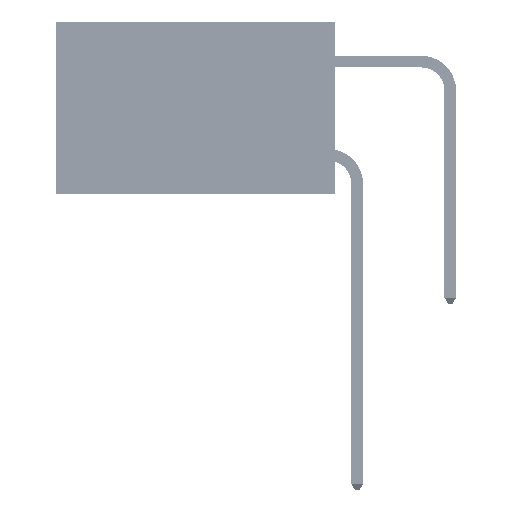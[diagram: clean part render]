
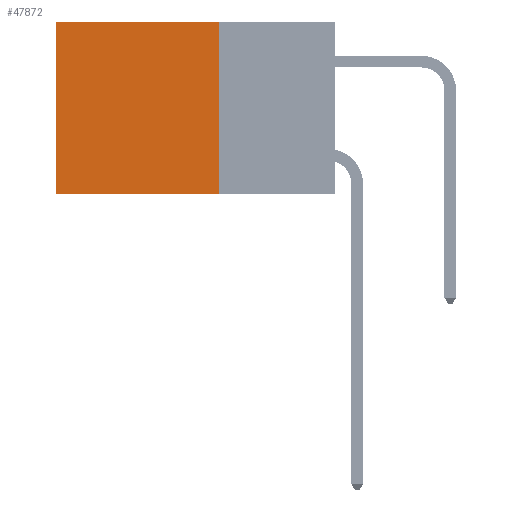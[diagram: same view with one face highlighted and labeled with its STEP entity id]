
A CAD part, left-side view. The second image highlights one B-rep face of the part: STEP entity #47872.
In plain terms, the highlighted planar face has unit normal (-1, 0, 0).
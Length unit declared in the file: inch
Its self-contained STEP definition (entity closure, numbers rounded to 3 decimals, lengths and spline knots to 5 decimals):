
#1948 = EDGE_LOOP ( 'NONE', ( #12003, #26524, #12206, #8017 ) ) ;
#1990 = EDGE_CURVE ( 'NONE', #3346, #23484, #13101, .T. ) ;
#3169 = LINE ( 'NONE', #30587, #11888 ) ;
#3346 = VERTEX_POINT ( 'NONE', #29523 ) ;
#7637 = VECTOR ( 'NONE', #46499, 39.37008 ) ;
#7987 = DIRECTION ( 'NONE',  ( 0., 1., 0. ) ) ;
#8017 = ORIENTED_EDGE ( 'NONE', *, *, #1990, .T. ) ;
#10217 = AXIS2_PLACEMENT_3D ( 'NONE', #22025, #18167, #44139 ) ;
#10958 = LINE ( 'NONE', #30447, #37101 ) ;
#11888 = VECTOR ( 'NONE', #19521, 39.37008 ) ;
#12003 = ORIENTED_EDGE ( 'NONE', *, *, #26641, .T. ) ;
#12206 = ORIENTED_EDGE ( 'NONE', *, *, #18746, .F. ) ;
#13101 = LINE ( 'NONE', #21629, #29981 ) ;
#15217 = PLANE ( 'NONE',  #10217 ) ;
#18167 = DIRECTION ( 'NONE',  ( 1., 0., 0. ) ) ;
#18746 = EDGE_CURVE ( 'NONE', #3346, #28924, #3169, .T. ) ;
#19151 = CARTESIAN_POINT ( 'NONE',  ( 0.2875, 0.6, -0.37 ) ) ;
#19521 = DIRECTION ( 'NONE',  ( 0., 0., -1. ) ) ;
#21226 = EDGE_CURVE ( 'NONE', #28924, #43679, #10958, .T. ) ;
#21629 = CARTESIAN_POINT ( 'NONE',  ( 0.2875, 0.25, 0. ) ) ;
#22025 = CARTESIAN_POINT ( 'NONE',  ( 0.2875, 0.25, 0. ) ) ;
#23484 = VERTEX_POINT ( 'NONE', #39138 ) ;
#24898 = DIRECTION ( 'NONE',  ( 0., 1., 0. ) ) ;
#26524 = ORIENTED_EDGE ( 'NONE', *, *, #21226, .F. ) ;
#26641 = EDGE_CURVE ( 'NONE', #23484, #43679, #27456, .T. ) ;
#27456 = LINE ( 'NONE', #31714, #7637 ) ;
#28924 = VERTEX_POINT ( 'NONE', #33060 ) ;
#29523 = CARTESIAN_POINT ( 'NONE',  ( 0.2875, 0.25, 0. ) ) ;
#29981 = VECTOR ( 'NONE', #24898, 39.37008 ) ;
#30447 = CARTESIAN_POINT ( 'NONE',  ( 0.2875, 0.25, -0.37 ) ) ;
#30587 = CARTESIAN_POINT ( 'NONE',  ( 0.2875, 0.25, 0. ) ) ;
#31714 = CARTESIAN_POINT ( 'NONE',  ( 0.2875, 0.6, 0. ) ) ;
#33060 = CARTESIAN_POINT ( 'NONE',  ( 0.2875, 0.25, -0.37 ) ) ;
#37101 = VECTOR ( 'NONE', #7987, 39.37008 ) ;
#39138 = CARTESIAN_POINT ( 'NONE',  ( 0.2875, 0.6, 0. ) ) ;
#41448 = FACE_OUTER_BOUND ( 'NONE', #1948, .T. ) ;
#43679 = VERTEX_POINT ( 'NONE', #19151 ) ;
#44139 = DIRECTION ( 'NONE',  ( 0., 0., -1. ) ) ;
#46499 = DIRECTION ( 'NONE',  ( 0., 0., -1. ) ) ;
#47872 = ADVANCED_FACE ( 'NONE', ( #41448 ), #15217, .F. ) ;
